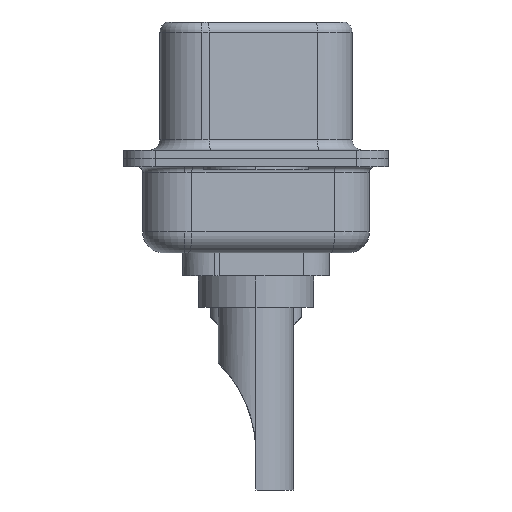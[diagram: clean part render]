
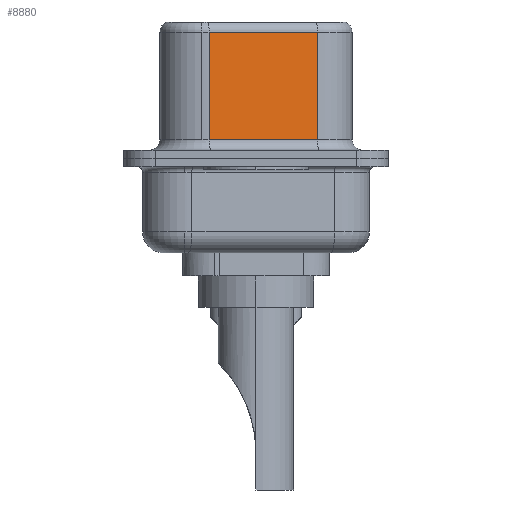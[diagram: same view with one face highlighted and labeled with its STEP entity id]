
A CAD part, left-side view. The second image highlights one B-rep face of the part: STEP entity #8880.
In plain terms, the highlighted planar face has unit normal (-0.985, -0.174, 0).
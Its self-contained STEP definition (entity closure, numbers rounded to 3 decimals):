
#825 = CARTESIAN_POINT ( 'NONE',  ( 4.565, -2.927, 6.02 ) ) ;
#1022 = ORIENTED_EDGE ( 'NONE', *, *, #14007, .T. ) ;
#1282 = ORIENTED_EDGE ( 'NONE', *, *, #11757, .F. ) ;
#1484 = CARTESIAN_POINT ( 'NONE',  ( 3.655, 2.233, 6.52 ) ) ;
#1600 = ORIENTED_EDGE ( 'NONE', *, *, #5193, .T. ) ;
#1949 = LINE ( 'NONE', #825, #4405 ) ;
#2736 = LINE ( 'NONE', #1484, #8540 ) ;
#3482 = VERTEX_POINT ( 'NONE', #5437 ) ;
#3494 = DIRECTION ( 'NONE',  ( 0., 0., -1. ) ) ;
#4405 = VECTOR ( 'NONE', #12134, 1000. ) ;
#4634 = FACE_OUTER_BOUND ( 'NONE', #8451, .T. ) ;
#5069 = CARTESIAN_POINT ( 'NONE',  ( 4.565, -2.927, 6.52 ) ) ;
#5086 = CARTESIAN_POINT ( 'NONE',  ( 4.565, -2.927, 6.02 ) ) ;
#5193 = EDGE_CURVE ( 'NONE', #12608, #10009, #1949, .T. ) ;
#5437 = CARTESIAN_POINT ( 'NONE',  ( 4.565, -2.927, 0.9 ) ) ;
#5884 = PLANE ( 'NONE',  #13015 ) ;
#5999 = DIRECTION ( 'NONE',  ( 0.174, -0.985, 0. ) ) ;
#7177 = LINE ( 'NONE', #13697, #12649 ) ;
#7699 = DIRECTION ( 'NONE',  ( 0.985, 0.174, 0. ) ) ;
#8012 = DIRECTION ( 'NONE',  ( 0., 0., -1. ) ) ;
#8451 = EDGE_LOOP ( 'NONE', ( #1282, #1600, #1022, #12206 ) ) ;
#8540 = VECTOR ( 'NONE', #8012, 1000. ) ;
#8880 = ADVANCED_FACE ( 'NONE', ( #4634 ), #5884, .F. ) ;
#8943 = LINE ( 'NONE', #11138, #12157 ) ;
#10009 = VERTEX_POINT ( 'NONE', #12191 ) ;
#10716 = VERTEX_POINT ( 'NONE', #13984 ) ;
#11138 = CARTESIAN_POINT ( 'NONE',  ( 4.565, -2.927, 6.52 ) ) ;
#11757 = EDGE_CURVE ( 'NONE', #12608, #3482, #8943, .T. ) ;
#12134 = DIRECTION ( 'NONE',  ( -0.174, 0.985, 0. ) ) ;
#12157 = VECTOR ( 'NONE', #3494, 1000. ) ;
#12191 = CARTESIAN_POINT ( 'NONE',  ( 3.655, 2.233, 6.02 ) ) ;
#12206 = ORIENTED_EDGE ( 'NONE', *, *, #12515, .T. ) ;
#12515 = EDGE_CURVE ( 'NONE', #10716, #3482, #7177, .T. ) ;
#12608 = VERTEX_POINT ( 'NONE', #5086 ) ;
#12649 = VECTOR ( 'NONE', #5999, 1000. ) ;
#13015 = AXIS2_PLACEMENT_3D ( 'NONE', #5069, #7699, #13683 ) ;
#13683 = DIRECTION ( 'NONE',  ( -0.174, 0.985, 0. ) ) ;
#13697 = CARTESIAN_POINT ( 'NONE',  ( 4.565, -2.927, 0.9 ) ) ;
#13984 = CARTESIAN_POINT ( 'NONE',  ( 3.655, 2.233, 0.9 ) ) ;
#14007 = EDGE_CURVE ( 'NONE', #10009, #10716, #2736, .T. ) ;
